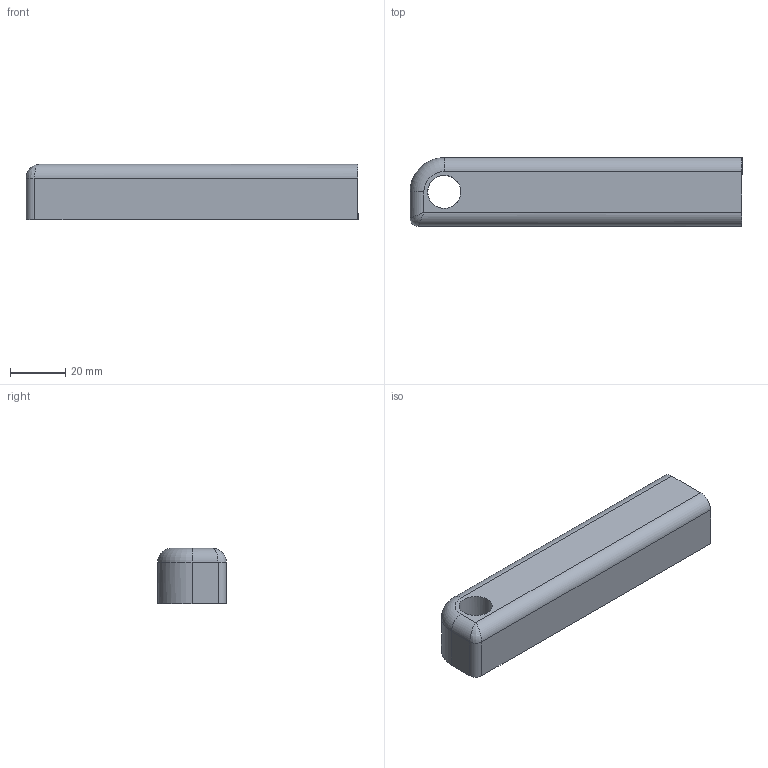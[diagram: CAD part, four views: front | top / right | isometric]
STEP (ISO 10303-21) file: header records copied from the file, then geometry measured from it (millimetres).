
FILE_DESCRIPTION (( 'STEP AP214' ), '1' );
FILE_NAME ('Bipod_Left_Part_2_V2.step', '2016-01-25T18:17:12', ( 'WarFairy' ), ( '' ), 'SwSTEP 2.0', 'SolidWorks 2015', '' );
FILE_SCHEMA (( 'AUTOMOTIVE_DESIGN' ));
Length unit declared in the file: millimetre
Products named in the file (1): Bipod_Left_Part_2_V2
Bounding box: 120 x 24.8 x 20 mm (x, y, z)
Volume: 54912.8 mm3; surface area: 11588.5 mm2
Topology: 1 solids, 1 shells, 50 faces, 140 edges, 79 vertices
Faces by surface type: cylinder 20, sphere 12, torus 10, plane 7, bspline 1
Full cylindrical faces by diameter (mm): 12 x1
Entity records: 1601 total; most frequent: CARTESIAN_POINT 394, DIRECTION 264, ORIENTED_EDGE 240, EDGE_CURVE 120, AXIS2_PLACEMENT_3D 113, VERTEX_POINT 73, CIRCLE 63, EDGE_LOOP 53
